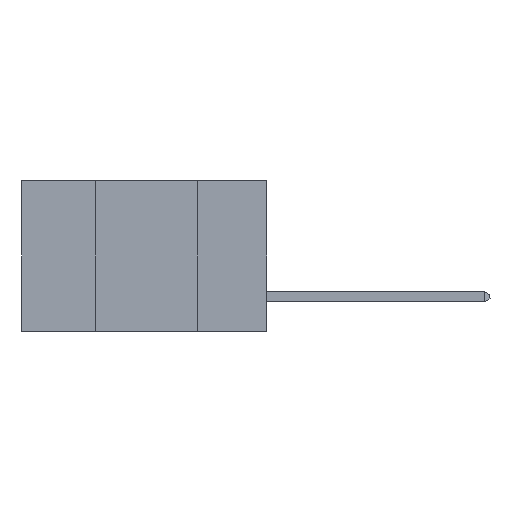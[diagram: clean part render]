
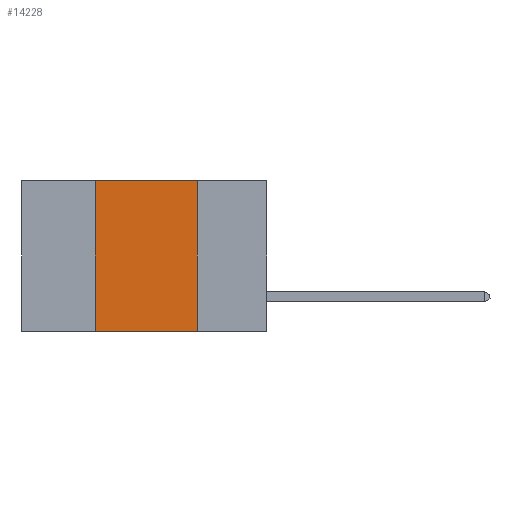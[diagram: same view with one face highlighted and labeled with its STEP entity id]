
A CAD part, left-side view. The second image highlights one B-rep face of the part: STEP entity #14228.
In plain terms, the highlighted planar face has unit normal (-1, 0, 0).
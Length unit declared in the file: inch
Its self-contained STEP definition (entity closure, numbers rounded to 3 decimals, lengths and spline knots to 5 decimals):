
#305 = CARTESIAN_POINT ( 'NONE',  ( 0., 0.42, 0. ) ) ;
#1445 = EDGE_CURVE ( 'NONE', #24145, #3917, #8323, .T. ) ;
#2229 = FACE_OUTER_BOUND ( 'NONE', #2860, .T. ) ;
#2366 = ORIENTED_EDGE ( 'NONE', *, *, #25540, .F. ) ;
#2705 = VERTEX_POINT ( 'NONE', #24878 ) ;
#2837 = VECTOR ( 'NONE', #4481, 39.37008 ) ;
#2860 = EDGE_LOOP ( 'NONE', ( #11987, #2366, #3666, #6923 ) ) ;
#3666 = ORIENTED_EDGE ( 'NONE', *, *, #1445, .F. ) ;
#3832 = LINE ( 'NONE', #8854, #19330 ) ;
#3917 = VERTEX_POINT ( 'NONE', #13377 ) ;
#4481 = DIRECTION ( 'NONE',  ( 0., 0., 1. ) ) ;
#5255 = CARTESIAN_POINT ( 'NONE',  ( 0., 0.17, 0. ) ) ;
#5490 = CARTESIAN_POINT ( 'NONE',  ( 0., 0.6, 0. ) ) ;
#5734 = EDGE_CURVE ( 'NONE', #24791, #2705, #3832, .T. ) ;
#6923 = ORIENTED_EDGE ( 'NONE', *, *, #12313, .T. ) ;
#8323 = LINE ( 'NONE', #305, #2837 ) ;
#8854 = CARTESIAN_POINT ( 'NONE',  ( 0., 0.17, 0. ) ) ;
#9984 = CARTESIAN_POINT ( 'NONE',  ( 0., 0.6, -0.37 ) ) ;
#10178 = CARTESIAN_POINT ( 'NONE',  ( 0., 0.6, 0. ) ) ;
#10992 = AXIS2_PLACEMENT_3D ( 'NONE', #10178, #16221, #12208 ) ;
#11987 = ORIENTED_EDGE ( 'NONE', *, *, #5734, .F. ) ;
#12208 = DIRECTION ( 'NONE',  ( 0., 0., -1. ) ) ;
#12313 = EDGE_CURVE ( 'NONE', #24145, #2705, #17857, .T. ) ;
#13377 = CARTESIAN_POINT ( 'NONE',  ( 0., 0.42, 0. ) ) ;
#14228 = ADVANCED_FACE ( 'NONE', ( #2229 ), #22150, .F. ) ;
#16221 = DIRECTION ( 'NONE',  ( 1., 0., 0. ) ) ;
#17857 = LINE ( 'NONE', #9984, #18479 ) ;
#18479 = VECTOR ( 'NONE', #23960, 39.37008 ) ;
#19330 = VECTOR ( 'NONE', #20861, 39.37008 ) ;
#19970 = LINE ( 'NONE', #5490, #25245 ) ;
#20861 = DIRECTION ( 'NONE',  ( 0., 0., -1. ) ) ;
#22150 = PLANE ( 'NONE',  #10992 ) ;
#23276 = CARTESIAN_POINT ( 'NONE',  ( 0., 0.42, -0.37 ) ) ;
#23299 = DIRECTION ( 'NONE',  ( 0., -1., 0. ) ) ;
#23960 = DIRECTION ( 'NONE',  ( 0., -1., 0. ) ) ;
#24145 = VERTEX_POINT ( 'NONE', #23276 ) ;
#24791 = VERTEX_POINT ( 'NONE', #5255 ) ;
#24878 = CARTESIAN_POINT ( 'NONE',  ( 0., 0.17, -0.37 ) ) ;
#25245 = VECTOR ( 'NONE', #23299, 39.37008 ) ;
#25540 = EDGE_CURVE ( 'NONE', #3917, #24791, #19970, .T. ) ;
